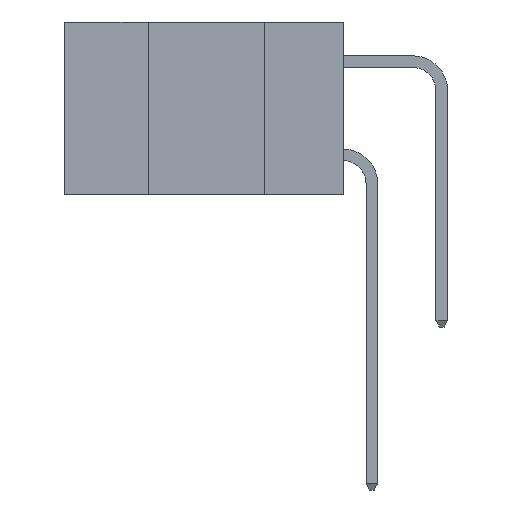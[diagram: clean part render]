
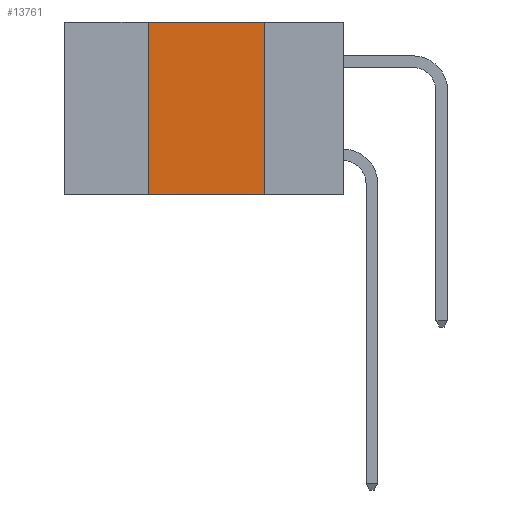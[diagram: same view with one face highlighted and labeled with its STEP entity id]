
A CAD part, left-side view. The second image highlights one B-rep face of the part: STEP entity #13761.
In plain terms, the highlighted planar face has unit normal (-1, 0, 0).
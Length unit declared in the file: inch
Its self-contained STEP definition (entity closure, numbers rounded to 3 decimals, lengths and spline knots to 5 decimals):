
#267 = VERTEX_POINT ( 'NONE', #5024 ) ;
#475 = CARTESIAN_POINT ( 'NONE',  ( 0., 0.6, 0. ) ) ;
#867 = VERTEX_POINT ( 'NONE', #13798 ) ;
#1152 = CARTESIAN_POINT ( 'NONE',  ( 0., 0.17, 0. ) ) ;
#1659 = CARTESIAN_POINT ( 'NONE',  ( 0., 0.42, -0.37 ) ) ;
#2004 = EDGE_CURVE ( 'NONE', #867, #7519, #6766, .T. ) ;
#2235 = FACE_OUTER_BOUND ( 'NONE', #8694, .T. ) ;
#2579 = LINE ( 'NONE', #1659, #11405 ) ;
#2734 = EDGE_CURVE ( 'NONE', #867, #267, #2579, .T. ) ;
#3221 = VECTOR ( 'NONE', #13086, 39.37008 ) ;
#3489 = EDGE_CURVE ( 'NONE', #267, #10925, #4965, .T. ) ;
#3821 = DIRECTION ( 'NONE',  ( 1., 0., 0. ) ) ;
#4934 = DIRECTION ( 'NONE',  ( 0., -1., 0. ) ) ;
#4948 = EDGE_CURVE ( 'NONE', #10925, #7519, #9422, .T. ) ;
#4965 = LINE ( 'NONE', #9339, #13381 ) ;
#5024 = CARTESIAN_POINT ( 'NONE',  ( 0., 0.42, 0. ) ) ;
#5491 = ORIENTED_EDGE ( 'NONE', *, *, #4948, .F. ) ;
#5642 = ORIENTED_EDGE ( 'NONE', *, *, #3489, .F. ) ;
#5675 = ORIENTED_EDGE ( 'NONE', *, *, #2734, .F. ) ;
#5870 = ORIENTED_EDGE ( 'NONE', *, *, #2004, .T. ) ;
#6423 = VECTOR ( 'NONE', #9198, 39.37008 ) ;
#6766 = LINE ( 'NONE', #10331, #6423 ) ;
#7519 = VERTEX_POINT ( 'NONE', #14198 ) ;
#8694 = EDGE_LOOP ( 'NONE', ( #5491, #5642, #5675, #5870 ) ) ;
#9198 = DIRECTION ( 'NONE',  ( 0., -1., 0. ) ) ;
#9339 = CARTESIAN_POINT ( 'NONE',  ( 0., 0.6, 0. ) ) ;
#9373 = DIRECTION ( 'NONE',  ( 0., 0., 1. ) ) ;
#9422 = LINE ( 'NONE', #10927, #3221 ) ;
#10331 = CARTESIAN_POINT ( 'NONE',  ( 0., 0.6, -0.37 ) ) ;
#10925 = VERTEX_POINT ( 'NONE', #1152 ) ;
#10927 = CARTESIAN_POINT ( 'NONE',  ( 0., 0.17, -0.37 ) ) ;
#11405 = VECTOR ( 'NONE', #9373, 39.37008 ) ;
#11542 = DIRECTION ( 'NONE',  ( 0., 0., -1. ) ) ;
#12563 = PLANE ( 'NONE',  #13427 ) ;
#13086 = DIRECTION ( 'NONE',  ( 0., 0., -1. ) ) ;
#13381 = VECTOR ( 'NONE', #4934, 39.37008 ) ;
#13427 = AXIS2_PLACEMENT_3D ( 'NONE', #475, #3821, #11542 ) ;
#13761 = ADVANCED_FACE ( 'NONE', ( #2235 ), #12563, .F. ) ;
#13798 = CARTESIAN_POINT ( 'NONE',  ( 0., 0.42, -0.37 ) ) ;
#14198 = CARTESIAN_POINT ( 'NONE',  ( 0., 0.17, -0.37 ) ) ;
